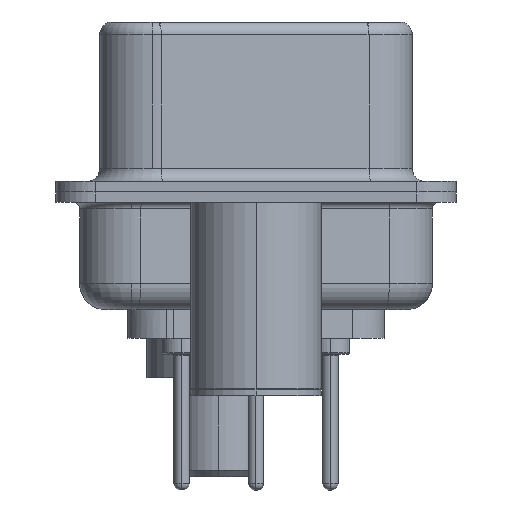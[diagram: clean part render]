
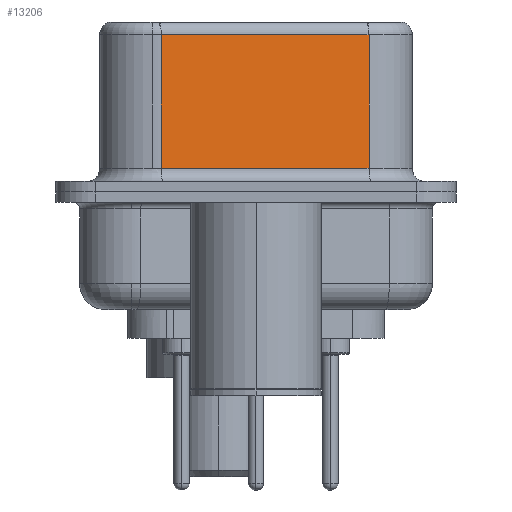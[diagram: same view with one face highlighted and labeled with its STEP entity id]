
A CAD part, left-side view. The second image highlights one B-rep face of the part: STEP entity #13206.
In plain terms, the highlighted planar face has unit normal (-0.985, -0.174, 0).
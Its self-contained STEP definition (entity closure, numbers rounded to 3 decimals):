
#301 = DIRECTION ( 'NONE',  ( -0.174, 0.985, 0. ) ) ;
#709 = VECTOR ( 'NONE', #1212, 1000. ) ;
#1212 = DIRECTION ( 'NONE',  ( 0., 0., -1. ) ) ;
#1698 = LINE ( 'NONE', #4453, #24755 ) ;
#2399 = PLANE ( 'NONE',  #15420 ) ;
#2482 = DIRECTION ( 'NONE',  ( 0.985, 0.174, 0. ) ) ;
#4453 = CARTESIAN_POINT ( 'NONE',  ( 5.132, -4.322, 6.52 ) ) ;
#7152 = EDGE_CURVE ( 'NONE', #18126, #15669, #8626, .T. ) ;
#7338 = LINE ( 'NONE', #14863, #13300 ) ;
#8352 = CARTESIAN_POINT ( 'NONE',  ( 5.132, -4.322, 6.02 ) ) ;
#8626 = LINE ( 'NONE', #18114, #13853 ) ;
#8832 = DIRECTION ( 'NONE',  ( 0., 0., -1. ) ) ;
#10940 = ORIENTED_EDGE ( 'NONE', *, *, #7152, .T. ) ;
#12113 = ORIENTED_EDGE ( 'NONE', *, *, #16491, .F. ) ;
#12314 = CARTESIAN_POINT ( 'NONE',  ( 3.73, 3.628, 6.52 ) ) ;
#12557 = LINE ( 'NONE', #12314, #709 ) ;
#12619 = DIRECTION ( 'NONE',  ( 0.174, -0.985, 0. ) ) ;
#13206 = ADVANCED_FACE ( 'NONE', ( #15488 ), #2399, .F. ) ;
#13300 = VECTOR ( 'NONE', #12619, 1000. ) ;
#13853 = VECTOR ( 'NONE', #301, 1000. ) ;
#14863 = CARTESIAN_POINT ( 'NONE',  ( 5.132, -4.322, 0.9 ) ) ;
#14954 = EDGE_CURVE ( 'NONE', #16754, #19104, #7338, .T. ) ;
#15420 = AXIS2_PLACEMENT_3D ( 'NONE', #24742, #2482, #18135 ) ;
#15488 = FACE_OUTER_BOUND ( 'NONE', #16228, .T. ) ;
#15669 = VERTEX_POINT ( 'NONE', #17509 ) ;
#15950 = EDGE_CURVE ( 'NONE', #15669, #16754, #12557, .T. ) ;
#16228 = EDGE_LOOP ( 'NONE', ( #12113, #10940, #18322, #28573 ) ) ;
#16373 = CARTESIAN_POINT ( 'NONE',  ( 5.132, -4.322, 0.9 ) ) ;
#16491 = EDGE_CURVE ( 'NONE', #18126, #19104, #1698, .T. ) ;
#16754 = VERTEX_POINT ( 'NONE', #27603 ) ;
#17509 = CARTESIAN_POINT ( 'NONE',  ( 3.73, 3.628, 6.02 ) ) ;
#18114 = CARTESIAN_POINT ( 'NONE',  ( 5.132, -4.322, 6.02 ) ) ;
#18126 = VERTEX_POINT ( 'NONE', #8352 ) ;
#18135 = DIRECTION ( 'NONE',  ( -0.174, 0.985, 0. ) ) ;
#18322 = ORIENTED_EDGE ( 'NONE', *, *, #15950, .T. ) ;
#19104 = VERTEX_POINT ( 'NONE', #16373 ) ;
#24742 = CARTESIAN_POINT ( 'NONE',  ( 5.132, -4.322, 6.52 ) ) ;
#24755 = VECTOR ( 'NONE', #8832, 1000. ) ;
#27603 = CARTESIAN_POINT ( 'NONE',  ( 3.73, 3.628, 0.9 ) ) ;
#28573 = ORIENTED_EDGE ( 'NONE', *, *, #14954, .T. ) ;
